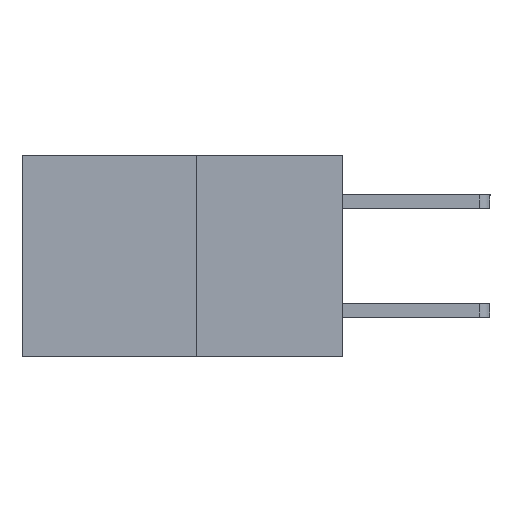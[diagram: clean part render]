
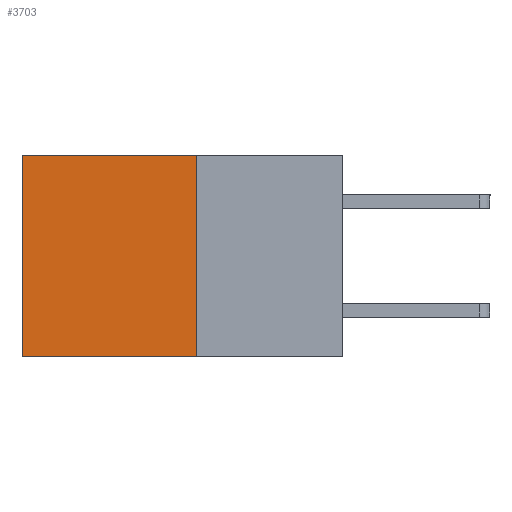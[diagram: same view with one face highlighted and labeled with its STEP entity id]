
A CAD part, left-side view. The second image highlights one B-rep face of the part: STEP entity #3703.
In plain terms, the highlighted planar face has unit normal (-1, 0, 0).
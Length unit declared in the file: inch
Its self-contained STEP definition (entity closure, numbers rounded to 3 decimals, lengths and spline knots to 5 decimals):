
#781 = CARTESIAN_POINT ( 'NONE',  ( 0.277, 0.27, -0.37 ) ) ;
#942 = LINE ( 'NONE', #5462, #2639 ) ;
#1053 = CARTESIAN_POINT ( 'NONE',  ( 0.277, 0.27, 0. ) ) ;
#1211 = LINE ( 'NONE', #4016, #5316 ) ;
#1350 = VERTEX_POINT ( 'NONE', #5250 ) ;
#1804 = VECTOR ( 'NONE', #9419, 39.37008 ) ;
#2639 = VECTOR ( 'NONE', #3828, 39.37008 ) ;
#2684 = EDGE_CURVE ( 'NONE', #1350, #6667, #9758, .T. ) ;
#3215 = DIRECTION ( 'NONE',  ( 0., 0., -1. ) ) ;
#3549 = CARTESIAN_POINT ( 'NONE',  ( 0.277, 0.59, -0.37 ) ) ;
#3703 = ADVANCED_FACE ( 'NONE', ( #4962 ), #7319, .F. ) ;
#3809 = ORIENTED_EDGE ( 'NONE', *, *, #2684, .T. ) ;
#3828 = DIRECTION ( 'NONE',  ( 0., 1., 0. ) ) ;
#4016 = CARTESIAN_POINT ( 'NONE',  ( 0.277, 0.27, -0.37 ) ) ;
#4404 = VERTEX_POINT ( 'NONE', #7593 ) ;
#4600 = CARTESIAN_POINT ( 'NONE',  ( 0.277, 0.27, -0.37 ) ) ;
#4800 = EDGE_CURVE ( 'NONE', #7473, #4404, #1211, .T. ) ;
#4920 = DIRECTION ( 'NONE',  ( 0., 0., -1. ) ) ;
#4962 = FACE_OUTER_BOUND ( 'NONE', #10270, .T. ) ;
#5250 = CARTESIAN_POINT ( 'NONE',  ( 0.277, 0.59, 0. ) ) ;
#5316 = VECTOR ( 'NONE', #3215, 39.37008 ) ;
#5345 = EDGE_CURVE ( 'NONE', #7473, #1350, #942, .T. ) ;
#5462 = CARTESIAN_POINT ( 'NONE',  ( 0.277, 0.27, 0. ) ) ;
#5502 = VECTOR ( 'NONE', #6955, 39.37008 ) ;
#5641 = ORIENTED_EDGE ( 'NONE', *, *, #4800, .F. ) ;
#5731 = ORIENTED_EDGE ( 'NONE', *, *, #5345, .T. ) ;
#6667 = VERTEX_POINT ( 'NONE', #9782 ) ;
#6718 = AXIS2_PLACEMENT_3D ( 'NONE', #781, #9732, #4920 ) ;
#6955 = DIRECTION ( 'NONE',  ( 0., 0., -1. ) ) ;
#7319 = PLANE ( 'NONE',  #6718 ) ;
#7473 = VERTEX_POINT ( 'NONE', #1053 ) ;
#7593 = CARTESIAN_POINT ( 'NONE',  ( 0.277, 0.27, -0.37 ) ) ;
#7682 = EDGE_CURVE ( 'NONE', #4404, #6667, #8034, .T. ) ;
#8034 = LINE ( 'NONE', #4600, #1804 ) ;
#8581 = ORIENTED_EDGE ( 'NONE', *, *, #7682, .F. ) ;
#9419 = DIRECTION ( 'NONE',  ( 0., 1., 0. ) ) ;
#9732 = DIRECTION ( 'NONE',  ( 1., 0., 0. ) ) ;
#9758 = LINE ( 'NONE', #3549, #5502 ) ;
#9782 = CARTESIAN_POINT ( 'NONE',  ( 0.277, 0.59, -0.37 ) ) ;
#10270 = EDGE_LOOP ( 'NONE', ( #3809, #8581, #5641, #5731 ) ) ;
